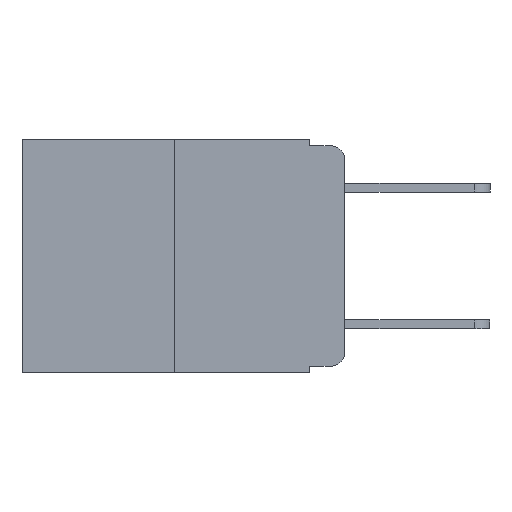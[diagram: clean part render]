
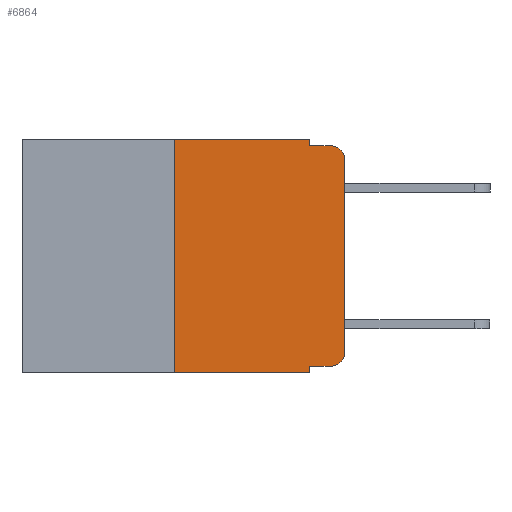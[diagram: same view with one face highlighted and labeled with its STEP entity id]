
A CAD part, left-side view. The second image highlights one B-rep face of the part: STEP entity #6864.
In plain terms, the highlighted planar face has unit normal (-1, 0, 0).
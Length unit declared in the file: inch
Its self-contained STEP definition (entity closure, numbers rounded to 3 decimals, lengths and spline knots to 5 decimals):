
#681 = LINE ( 'NONE', #15723, #5145 ) ;
#1129 = CARTESIAN_POINT ( 'NONE',  ( 0., 0.25, 0. ) ) ;
#1218 = VECTOR ( 'NONE', #4253, 39.37008 ) ;
#1243 = EDGE_CURVE ( 'NONE', #3272, #9378, #3192, .T. ) ;
#1646 = VECTOR ( 'NONE', #11759, 39.37008 ) ;
#1890 = EDGE_CURVE ( 'NONE', #12509, #4192, #8378, .T. ) ;
#2093 = CIRCLE ( 'NONE', #8024, 0.02 ) ;
#2127 = PLANE ( 'NONE',  #4280 ) ;
#2567 = EDGE_CURVE ( 'NONE', #6230, #12178, #5578, .T. ) ;
#2570 = EDGE_CURVE ( 'NONE', #12178, #9382, #2093, .T. ) ;
#2594 = EDGE_CURVE ( 'NONE', #13866, #9382, #11520, .T. ) ;
#2600 = EDGE_CURVE ( 'NONE', #9378, #13866, #681, .T. ) ;
#2632 = EDGE_CURVE ( 'NONE', #12509, #3272, #14220, .T. ) ;
#2635 = EDGE_CURVE ( 'NONE', #14396, #4192, #11143, .T. ) ;
#2673 = EDGE_CURVE ( 'NONE', #14396, #9621, #10024, .T. ) ;
#2700 = EDGE_CURVE ( 'NONE', #9621, #6230, #12828, .T. ) ;
#3192 = LINE ( 'NONE', #14193, #9908 ) ;
#3272 = VERTEX_POINT ( 'NONE', #1129 ) ;
#3546 = CARTESIAN_POINT ( 'NONE',  ( 0., 0.473, -0.343 ) ) ;
#4132 = CARTESIAN_POINT ( 'NONE',  ( 0., 0.051, -0.333 ) ) ;
#4192 = VERTEX_POINT ( 'NONE', #7828 ) ;
#4253 = DIRECTION ( 'NONE',  ( 0., -1., 0. ) ) ;
#4280 = AXIS2_PLACEMENT_3D ( 'NONE', #7891, #16033, #9158 ) ;
#4799 = CARTESIAN_POINT ( 'NONE',  ( 0., 0.02, -0.03 ) ) ;
#4805 = CARTESIAN_POINT ( 'NONE',  ( 0., 0.02, -0.313 ) ) ;
#4898 = AXIS2_PLACEMENT_3D ( 'NONE', #4805, #5875, #5800 ) ;
#4973 = EDGE_LOOP ( 'NONE', ( #11192, #11291, #11473, #11488, #11625, #11658, #12164, #12281, #12378, #12596 ) ) ;
#5145 = VECTOR ( 'NONE', #14976, 39.37008 ) ;
#5436 = DIRECTION ( 'NONE',  ( -1., 0., 0. ) ) ;
#5578 = LINE ( 'NONE', #15459, #1646 ) ;
#5800 = DIRECTION ( 'NONE',  ( 0., 0., -1. ) ) ;
#5875 = DIRECTION ( 'NONE',  ( -1., 0., 0. ) ) ;
#6230 = VERTEX_POINT ( 'NONE', #10674 ) ;
#6556 = DIRECTION ( 'NONE',  ( 0., -1., 0. ) ) ;
#6864 = ADVANCED_FACE ( 'NONE', ( #12406 ), #2127, .F. ) ;
#7828 = CARTESIAN_POINT ( 'NONE',  ( 0., 0.051, -0.343 ) ) ;
#7891 = CARTESIAN_POINT ( 'NONE',  ( 0., 0.473, 0. ) ) ;
#7929 = VECTOR ( 'NONE', #10915, 39.37008 ) ;
#8024 = AXIS2_PLACEMENT_3D ( 'NONE', #4799, #5436, #11597 ) ;
#8337 = VECTOR ( 'NONE', #6556, 39.37008 ) ;
#8378 = LINE ( 'NONE', #3546, #1218 ) ;
#9032 = CARTESIAN_POINT ( 'NONE',  ( 0., 0., -0.03 ) ) ;
#9158 = DIRECTION ( 'NONE',  ( 0., 0., -1. ) ) ;
#9378 = VERTEX_POINT ( 'NONE', #10975 ) ;
#9382 = VERTEX_POINT ( 'NONE', #9781 ) ;
#9621 = VERTEX_POINT ( 'NONE', #13528 ) ;
#9781 = CARTESIAN_POINT ( 'NONE',  ( 0., 0.02, -0.01 ) ) ;
#9908 = VECTOR ( 'NONE', #16583, 39.37008 ) ;
#10024 = LINE ( 'NONE', #13057, #13520 ) ;
#10656 = CARTESIAN_POINT ( 'NONE',  ( 0., 0.051, -0.01 ) ) ;
#10674 = CARTESIAN_POINT ( 'NONE',  ( 0., 0., -0.313 ) ) ;
#10915 = DIRECTION ( 'NONE',  ( 0., 0., -1. ) ) ;
#10975 = CARTESIAN_POINT ( 'NONE',  ( 0., 0.051, 0. ) ) ;
#11016 = CARTESIAN_POINT ( 'NONE',  ( 0., 0.051, 0. ) ) ;
#11143 = LINE ( 'NONE', #11016, #7929 ) ;
#11192 = ORIENTED_EDGE ( 'NONE', *, *, #2567, .T. ) ;
#11291 = ORIENTED_EDGE ( 'NONE', *, *, #2570, .T. ) ;
#11473 = ORIENTED_EDGE ( 'NONE', *, *, #2594, .F. ) ;
#11488 = ORIENTED_EDGE ( 'NONE', *, *, #2600, .F. ) ;
#11520 = LINE ( 'NONE', #14840, #8337 ) ;
#11597 = DIRECTION ( 'NONE',  ( 0., 0., -1. ) ) ;
#11625 = ORIENTED_EDGE ( 'NONE', *, *, #1243, .F. ) ;
#11658 = ORIENTED_EDGE ( 'NONE', *, *, #2632, .F. ) ;
#11759 = DIRECTION ( 'NONE',  ( 0., 0., 1. ) ) ;
#12035 = DIRECTION ( 'NONE',  ( 0., 0., 1. ) ) ;
#12164 = ORIENTED_EDGE ( 'NONE', *, *, #1890, .T. ) ;
#12178 = VERTEX_POINT ( 'NONE', #9032 ) ;
#12281 = ORIENTED_EDGE ( 'NONE', *, *, #2635, .F. ) ;
#12378 = ORIENTED_EDGE ( 'NONE', *, *, #2673, .T. ) ;
#12406 = FACE_OUTER_BOUND ( 'NONE', #4973, .T. ) ;
#12509 = VERTEX_POINT ( 'NONE', #15105 ) ;
#12596 = ORIENTED_EDGE ( 'NONE', *, *, #2700, .T. ) ;
#12691 = DIRECTION ( 'NONE',  ( 0., -1., 0. ) ) ;
#12828 = CIRCLE ( 'NONE', #4898, 0.02 ) ;
#12840 = CARTESIAN_POINT ( 'NONE',  ( 0., 0.25, 0. ) ) ;
#13057 = CARTESIAN_POINT ( 'NONE',  ( 0., 0.051, -0.333 ) ) ;
#13520 = VECTOR ( 'NONE', #12691, 39.37008 ) ;
#13528 = CARTESIAN_POINT ( 'NONE',  ( 0., 0.02, -0.333 ) ) ;
#13864 = VECTOR ( 'NONE', #12035, 39.37008 ) ;
#13866 = VERTEX_POINT ( 'NONE', #10656 ) ;
#14193 = CARTESIAN_POINT ( 'NONE',  ( 0., 0.473, 0. ) ) ;
#14220 = LINE ( 'NONE', #12840, #13864 ) ;
#14396 = VERTEX_POINT ( 'NONE', #4132 ) ;
#14840 = CARTESIAN_POINT ( 'NONE',  ( 0., 0.051, -0.01 ) ) ;
#14976 = DIRECTION ( 'NONE',  ( 0., 0., -1. ) ) ;
#15105 = CARTESIAN_POINT ( 'NONE',  ( 0., 0.25, -0.343 ) ) ;
#15459 = CARTESIAN_POINT ( 'NONE',  ( 0., 0., 0. ) ) ;
#15723 = CARTESIAN_POINT ( 'NONE',  ( 0., 0.051, 0. ) ) ;
#16033 = DIRECTION ( 'NONE',  ( 1., 0., 0. ) ) ;
#16583 = DIRECTION ( 'NONE',  ( 0., -1., 0. ) ) ;
